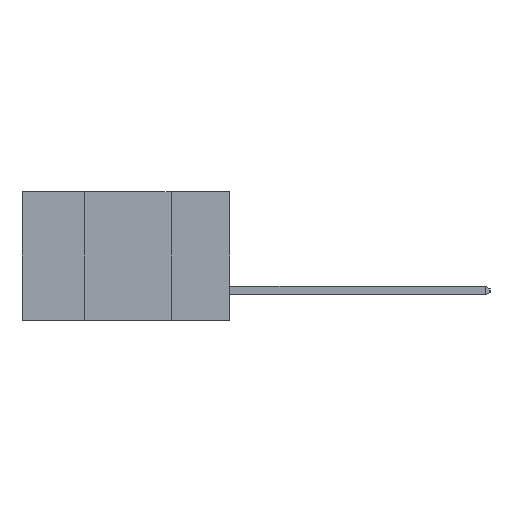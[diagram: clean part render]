
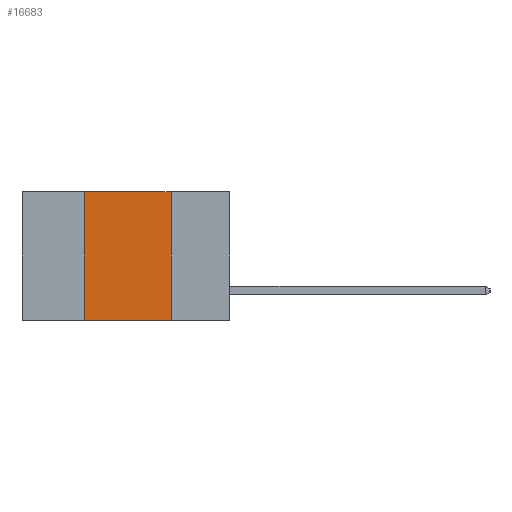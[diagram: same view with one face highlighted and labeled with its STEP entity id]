
A CAD part, left-side view. The second image highlights one B-rep face of the part: STEP entity #16683.
In plain terms, the highlighted planar face has unit normal (-1, 0, 0).
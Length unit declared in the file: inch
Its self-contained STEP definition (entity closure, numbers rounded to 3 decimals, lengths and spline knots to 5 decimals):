
#748 = DIRECTION ( 'NONE',  ( 0., 0., -1. ) ) ;
#809 = VECTOR ( 'NONE', #3900, 39.37008 ) ;
#886 = DIRECTION ( 'NONE',  ( 0., -1., 0. ) ) ;
#890 = DIRECTION ( 'NONE',  ( 0., 0., -1. ) ) ;
#1105 = VERTEX_POINT ( 'NONE', #19783 ) ;
#3900 = DIRECTION ( 'NONE',  ( 0., 0., 1. ) ) ;
#3942 = ORIENTED_EDGE ( 'NONE', *, *, #23459, .T. ) ;
#4933 = LINE ( 'NONE', #20511, #27867 ) ;
#5257 = CARTESIAN_POINT ( 'NONE',  ( 0., 0.42, -0.37 ) ) ;
#5947 = VECTOR ( 'NONE', #890, 39.37008 ) ;
#7001 = CARTESIAN_POINT ( 'NONE',  ( 0., 0.42, 0. ) ) ;
#7357 = PLANE ( 'NONE',  #25106 ) ;
#7850 = CARTESIAN_POINT ( 'NONE',  ( 0., 0.17, 0. ) ) ;
#7997 = VERTEX_POINT ( 'NONE', #7001 ) ;
#8677 = CARTESIAN_POINT ( 'NONE',  ( 0., 0.6, -0.37 ) ) ;
#8882 = LINE ( 'NONE', #8677, #24704 ) ;
#10628 = EDGE_LOOP ( 'NONE', ( #17230, #24249, #20560, #3942 ) ) ;
#10888 = DIRECTION ( 'NONE',  ( 0., -1., 0. ) ) ;
#11554 = EDGE_CURVE ( 'NONE', #7997, #26904, #4933, .T. ) ;
#12675 = CARTESIAN_POINT ( 'NONE',  ( 0., 0.42, 0. ) ) ;
#13444 = EDGE_CURVE ( 'NONE', #26904, #1105, #22521, .T. ) ;
#13968 = DIRECTION ( 'NONE',  ( 1., 0., 0. ) ) ;
#14102 = CARTESIAN_POINT ( 'NONE',  ( 0., 0.17, 0. ) ) ;
#16683 = ADVANCED_FACE ( 'NONE', ( #19338 ), #7357, .F. ) ;
#17230 = ORIENTED_EDGE ( 'NONE', *, *, #13444, .F. ) ;
#17728 = EDGE_CURVE ( 'NONE', #24254, #7997, #23953, .T. ) ;
#19338 = FACE_OUTER_BOUND ( 'NONE', #10628, .T. ) ;
#19783 = CARTESIAN_POINT ( 'NONE',  ( 0., 0.17, -0.37 ) ) ;
#20511 = CARTESIAN_POINT ( 'NONE',  ( 0., 0.6, 0. ) ) ;
#20560 = ORIENTED_EDGE ( 'NONE', *, *, #17728, .F. ) ;
#22521 = LINE ( 'NONE', #14102, #5947 ) ;
#23459 = EDGE_CURVE ( 'NONE', #24254, #1105, #8882, .T. ) ;
#23953 = LINE ( 'NONE', #12675, #809 ) ;
#24249 = ORIENTED_EDGE ( 'NONE', *, *, #11554, .F. ) ;
#24254 = VERTEX_POINT ( 'NONE', #5257 ) ;
#24704 = VECTOR ( 'NONE', #10888, 39.37008 ) ;
#25106 = AXIS2_PLACEMENT_3D ( 'NONE', #26745, #13968, #748 ) ;
#26745 = CARTESIAN_POINT ( 'NONE',  ( 0., 0.6, 0. ) ) ;
#26904 = VERTEX_POINT ( 'NONE', #7850 ) ;
#27867 = VECTOR ( 'NONE', #886, 39.37008 ) ;
